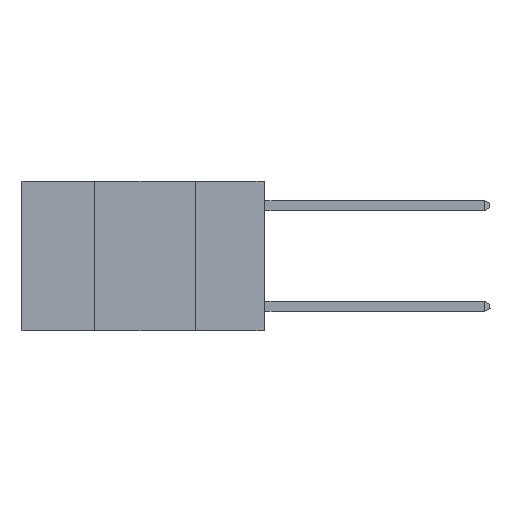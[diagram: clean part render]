
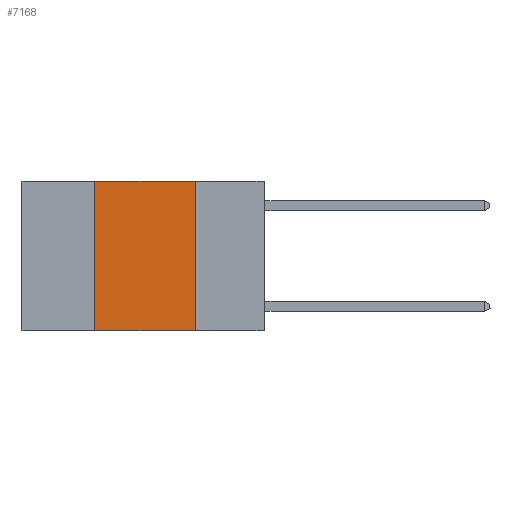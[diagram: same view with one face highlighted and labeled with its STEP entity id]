
A CAD part, left-side view. The second image highlights one B-rep face of the part: STEP entity #7168.
In plain terms, the highlighted planar face has unit normal (-1, 0, 0).
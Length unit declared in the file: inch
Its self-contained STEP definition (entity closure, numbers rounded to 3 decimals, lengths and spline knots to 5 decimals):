
#205 = VECTOR ( 'NONE', #6037, 39.37008 ) ;
#438 = EDGE_CURVE ( 'NONE', #6910, #3582, #6491, .T. ) ;
#1424 = VERTEX_POINT ( 'NONE', #6123 ) ;
#1425 = CARTESIAN_POINT ( 'NONE',  ( 0., 0.17, 0. ) ) ;
#1569 = DIRECTION ( 'NONE',  ( 0., -1., 0. ) ) ;
#1595 = CARTESIAN_POINT ( 'NONE',  ( 0., 0.6, 0. ) ) ;
#1817 = DIRECTION ( 'NONE',  ( 0., 0., -1. ) ) ;
#2075 = CARTESIAN_POINT ( 'NONE',  ( 0., 0.6, -0.37 ) ) ;
#2233 = FACE_OUTER_BOUND ( 'NONE', #6165, .T. ) ;
#2238 = ORIENTED_EDGE ( 'NONE', *, *, #4600, .T. ) ;
#2304 = VECTOR ( 'NONE', #3269, 39.37008 ) ;
#3269 = DIRECTION ( 'NONE',  ( 0., 0., -1. ) ) ;
#3345 = CARTESIAN_POINT ( 'NONE',  ( 0., 0.17, 0. ) ) ;
#3476 = LINE ( 'NONE', #4077, #205 ) ;
#3500 = CARTESIAN_POINT ( 'NONE',  ( 0., 0.6, 0. ) ) ;
#3515 = AXIS2_PLACEMENT_3D ( 'NONE', #1595, #6873, #1817 ) ;
#3582 = VERTEX_POINT ( 'NONE', #6368 ) ;
#3786 = ORIENTED_EDGE ( 'NONE', *, *, #3896, .F. ) ;
#3896 = EDGE_CURVE ( 'NONE', #5401, #6910, #4904, .T. ) ;
#4010 = CARTESIAN_POINT ( 'NONE',  ( 0., 0.42, 0. ) ) ;
#4077 = CARTESIAN_POINT ( 'NONE',  ( 0., 0.42, 0. ) ) ;
#4600 = EDGE_CURVE ( 'NONE', #1424, #3582, #6666, .T. ) ;
#4613 = EDGE_CURVE ( 'NONE', #1424, #5401, #3476, .T. ) ;
#4711 = DIRECTION ( 'NONE',  ( 0., -1., 0. ) ) ;
#4847 = PLANE ( 'NONE',  #3515 ) ;
#4904 = LINE ( 'NONE', #3500, #7529 ) ;
#5107 = ORIENTED_EDGE ( 'NONE', *, *, #4613, .F. ) ;
#5401 = VERTEX_POINT ( 'NONE', #4010 ) ;
#5547 = ORIENTED_EDGE ( 'NONE', *, *, #438, .F. ) ;
#6037 = DIRECTION ( 'NONE',  ( 0., 0., 1. ) ) ;
#6123 = CARTESIAN_POINT ( 'NONE',  ( 0., 0.42, -0.37 ) ) ;
#6165 = EDGE_LOOP ( 'NONE', ( #5547, #3786, #5107, #2238 ) ) ;
#6368 = CARTESIAN_POINT ( 'NONE',  ( 0., 0.17, -0.37 ) ) ;
#6491 = LINE ( 'NONE', #3345, #2304 ) ;
#6666 = LINE ( 'NONE', #2075, #8343 ) ;
#6873 = DIRECTION ( 'NONE',  ( 1., 0., 0. ) ) ;
#6910 = VERTEX_POINT ( 'NONE', #1425 ) ;
#7168 = ADVANCED_FACE ( 'NONE', ( #2233 ), #4847, .F. ) ;
#7529 = VECTOR ( 'NONE', #1569, 39.37008 ) ;
#8343 = VECTOR ( 'NONE', #4711, 39.37008 ) ;
